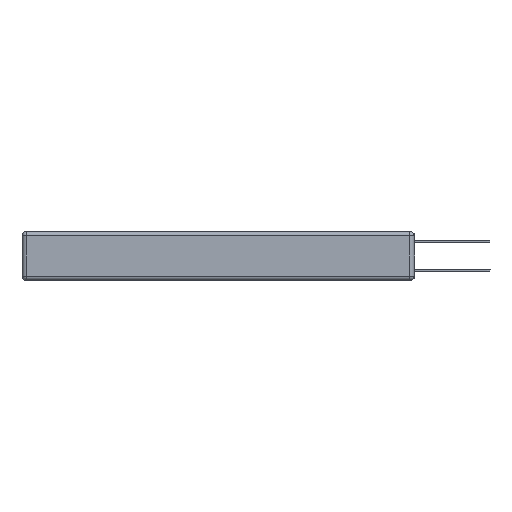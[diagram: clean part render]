
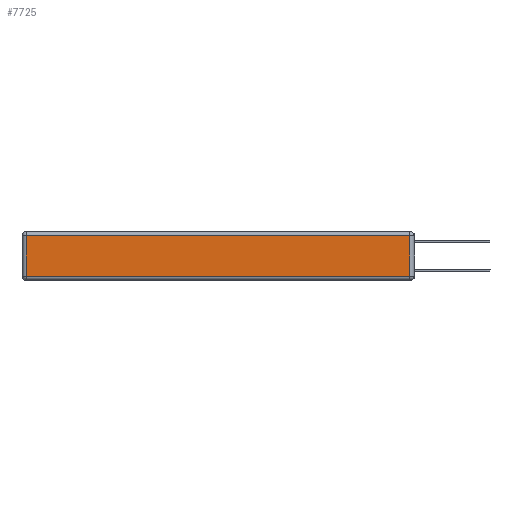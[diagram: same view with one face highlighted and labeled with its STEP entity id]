
A CAD part, left-side view. The second image highlights one B-rep face of the part: STEP entity #7725.
In plain terms, the highlighted planar face has unit normal (-1, 0, 0).
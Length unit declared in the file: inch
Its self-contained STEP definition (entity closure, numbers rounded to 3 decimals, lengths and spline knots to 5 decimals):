
#625 = EDGE_CURVE ( 'NONE', #8552, #833, #4452, .T. ) ;
#833 = VERTEX_POINT ( 'NONE', #7974 ) ;
#835 = VECTOR ( 'NONE', #10819, 39.37008 ) ;
#853 = ORIENTED_EDGE ( 'NONE', *, *, #5544, .T. ) ;
#1447 = CARTESIAN_POINT ( 'NONE',  ( 0., 2.72, -0.03 ) ) ;
#1929 = DIRECTION ( 'NONE',  ( 0., -1., 0. ) ) ;
#1964 = CARTESIAN_POINT ( 'NONE',  ( 0., 0.03, -0.03 ) ) ;
#2483 = VECTOR ( 'NONE', #1929, 39.37008 ) ;
#2583 = LINE ( 'NONE', #12047, #835 ) ;
#3783 = LINE ( 'NONE', #10848, #10319 ) ;
#3898 = ORIENTED_EDGE ( 'NONE', *, *, #5450, .T. ) ;
#4195 = DIRECTION ( 'NONE',  ( 0., 0., 1. ) ) ;
#4386 = VERTEX_POINT ( 'NONE', #1447 ) ;
#4452 = LINE ( 'NONE', #15436, #2483 ) ;
#4954 = LINE ( 'NONE', #14269, #7136 ) ;
#5450 = EDGE_CURVE ( 'NONE', #4386, #8552, #4954, .T. ) ;
#5468 = PLANE ( 'NONE',  #5808 ) ;
#5544 = EDGE_CURVE ( 'NONE', #833, #13717, #2583, .T. ) ;
#5808 = AXIS2_PLACEMENT_3D ( 'NONE', #11709, #7962, #4195 ) ;
#7136 = VECTOR ( 'NONE', #15646, 39.37008 ) ;
#7425 = EDGE_LOOP ( 'NONE', ( #14040, #853, #16311, #3898 ) ) ;
#7725 = ADVANCED_FACE ( 'NONE', ( #8046 ), #5468, .T. ) ;
#7962 = DIRECTION ( 'NONE',  ( -1., 0., 0. ) ) ;
#7974 = CARTESIAN_POINT ( 'NONE',  ( 0., 0.03, -0.313 ) ) ;
#8046 = FACE_OUTER_BOUND ( 'NONE', #7425, .T. ) ;
#8552 = VERTEX_POINT ( 'NONE', #11077 ) ;
#10319 = VECTOR ( 'NONE', #13464, 39.37008 ) ;
#10819 = DIRECTION ( 'NONE',  ( 0., 0., 1. ) ) ;
#10848 = CARTESIAN_POINT ( 'NONE',  ( 0., 2.75, -0.03 ) ) ;
#11077 = CARTESIAN_POINT ( 'NONE',  ( 0., 2.72, -0.313 ) ) ;
#11709 = CARTESIAN_POINT ( 'NONE',  ( 0., 0., -0.343 ) ) ;
#12047 = CARTESIAN_POINT ( 'NONE',  ( 0., 0.03, -0.343 ) ) ;
#12390 = EDGE_CURVE ( 'NONE', #13717, #4386, #3783, .T. ) ;
#13464 = DIRECTION ( 'NONE',  ( 0., 1., 0. ) ) ;
#13717 = VERTEX_POINT ( 'NONE', #1964 ) ;
#14040 = ORIENTED_EDGE ( 'NONE', *, *, #625, .T. ) ;
#14269 = CARTESIAN_POINT ( 'NONE',  ( 0., 2.72, -0.343 ) ) ;
#15436 = CARTESIAN_POINT ( 'NONE',  ( 0., 0., -0.313 ) ) ;
#15646 = DIRECTION ( 'NONE',  ( 0., 0., -1. ) ) ;
#16311 = ORIENTED_EDGE ( 'NONE', *, *, #12390, .T. ) ;
